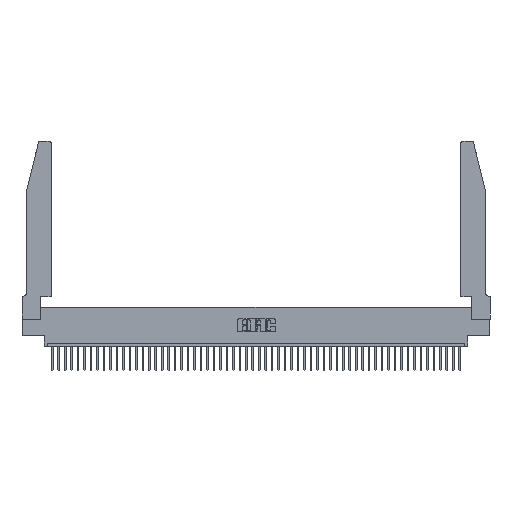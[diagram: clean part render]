
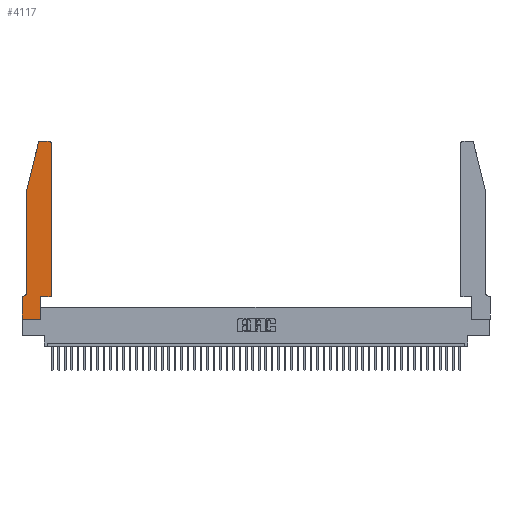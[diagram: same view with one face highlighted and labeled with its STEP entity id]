
A CAD part, top view. The second image highlights one B-rep face of the part: STEP entity #4117.
In plain terms, the highlighted planar face has unit normal (0, 0, 1).
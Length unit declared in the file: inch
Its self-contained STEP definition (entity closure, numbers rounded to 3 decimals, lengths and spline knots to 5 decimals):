
#409 = VERTEX_POINT ( 'NONE', #47005 ) ;
#2255 = CARTESIAN_POINT ( 'NONE',  ( 0.4505, 0.35, 0.37 ) ) ;
#2574 = FACE_OUTER_BOUND ( 'NONE', #24028, .T. ) ;
#3259 = CARTESIAN_POINT ( 'NONE',  ( 0.4205, 2.75, 0.37 ) ) ;
#3385 = CARTESIAN_POINT ( 'NONE',  ( 0.25487, 2.72718, 0.37 ) ) ;
#4117 = ADVANCED_FACE ( 'NONE', ( #2574 ), #21660, .T. ) ;
#5095 = ORIENTED_EDGE ( 'NONE', *, *, #29858, .T. ) ;
#5390 = ORIENTED_EDGE ( 'NONE', *, *, #9491, .T. ) ;
#6916 = ORIENTED_EDGE ( 'NONE', *, *, #14958, .T. ) ;
#8444 = VECTOR ( 'NONE', #34154, 39.37008 ) ;
#8892 = DIRECTION ( 'NONE',  ( 0., 1., 0. ) ) ;
#9297 = EDGE_CURVE ( 'NONE', #42854, #43902, #35068, .T. ) ;
#9491 = EDGE_CURVE ( 'NONE', #19205, #42175, #24732, .T. ) ;
#9789 = ORIENTED_EDGE ( 'NONE', *, *, #31108, .T. ) ;
#10030 = ORIENTED_EDGE ( 'NONE', *, *, #9297, .T. ) ;
#10309 = LINE ( 'NONE', #31914, #43622 ) ;
#10719 = VERTEX_POINT ( 'NONE', #40777 ) ;
#10902 = CARTESIAN_POINT ( 'NONE',  ( 0.284, 2.72, 0.37 ) ) ;
#12161 = LINE ( 'NONE', #43560, #28570 ) ;
#12295 = EDGE_CURVE ( 'NONE', #14741, #10719, #37264, .T. ) ;
#13896 = DIRECTION ( 'NONE',  ( -1., 0., 0. ) ) ;
#14625 = VERTEX_POINT ( 'NONE', #3385 ) ;
#14741 = VERTEX_POINT ( 'NONE', #3259 ) ;
#14958 = EDGE_CURVE ( 'NONE', #10719, #14625, #36955, .T. ) ;
#15342 = CARTESIAN_POINT ( 'NONE',  ( 0., 0., 0.37 ) ) ;
#17574 = LINE ( 'NONE', #41969, #8444 ) ;
#18045 = DIRECTION ( 'NONE',  ( 0., 0., -1. ) ) ;
#19205 = VERTEX_POINT ( 'NONE', #47621 ) ;
#19671 = CARTESIAN_POINT ( 'NONE',  ( 0.0055, 0.35, 0.37 ) ) ;
#20083 = ORIENTED_EDGE ( 'NONE', *, *, #25597, .T. ) ;
#20378 = CARTESIAN_POINT ( 'NONE',  ( 0.0755, 0.42, 0.37 ) ) ;
#21195 = ORIENTED_EDGE ( 'NONE', *, *, #40685, .T. ) ;
#21383 = CARTESIAN_POINT ( 'NONE',  ( 0.0755, 0.35, 0.37 ) ) ;
#21613 = DIRECTION ( 'NONE',  ( -1., 0., 0. ) ) ;
#21660 = PLANE ( 'NONE',  #45626 ) ;
#22224 = ORIENTED_EDGE ( 'NONE', *, *, #28083, .T. ) ;
#22719 = LINE ( 'NONE', #32537, #29141 ) ;
#23023 = EDGE_CURVE ( 'NONE', #14625, #31736, #22719, .T. ) ;
#24028 = EDGE_LOOP ( 'NONE', ( #38230, #6916, #30427, #21195, #20083, #10030, #5095, #38430, #22224, #5390, #9789, #43598 ) ) ;
#24732 = LINE ( 'NONE', #2255, #42411 ) ;
#24909 = CARTESIAN_POINT ( 'NONE',  ( 0.2865, 0.35, 0.37 ) ) ;
#25385 = DIRECTION ( 'NONE',  ( 0., 0., 1. ) ) ;
#25597 = EDGE_CURVE ( 'NONE', #33444, #42854, #49555, .T. ) ;
#25890 = AXIS2_PLACEMENT_3D ( 'NONE', #10902, #49863, #33615 ) ;
#26767 = CARTESIAN_POINT ( 'NONE',  ( 0.4505, 0.35, 0.37 ) ) ;
#28083 = EDGE_CURVE ( 'NONE', #409, #19205, #46859, .T. ) ;
#28570 = VECTOR ( 'NONE', #30235, 39.37008 ) ;
#28667 = DIRECTION ( 'NONE',  ( 0., 0., 1. ) ) ;
#28878 = EDGE_CURVE ( 'NONE', #40422, #14741, #29231, .T. ) ;
#29141 = VECTOR ( 'NONE', #32380, 39.37008 ) ;
#29231 = CIRCLE ( 'NONE', #36938, 0.03 ) ;
#29537 = CARTESIAN_POINT ( 'NONE',  ( 0.0055, 0.42, 0.37 ) ) ;
#29858 = EDGE_CURVE ( 'NONE', #43902, #39477, #12161, .T. ) ;
#29966 = VECTOR ( 'NONE', #49445, 39.37008 ) ;
#30235 = DIRECTION ( 'NONE',  ( 0., -1., 0. ) ) ;
#30427 = ORIENTED_EDGE ( 'NONE', *, *, #23023, .T. ) ;
#30443 = LINE ( 'NONE', #47049, #48540 ) ;
#31108 = EDGE_CURVE ( 'NONE', #42175, #40422, #10309, .T. ) ;
#31736 = VERTEX_POINT ( 'NONE', #37834 ) ;
#31805 = CARTESIAN_POINT ( 'NONE',  ( 0., 0.35, 0.37 ) ) ;
#31914 = CARTESIAN_POINT ( 'NONE',  ( 0.4505, 0.35, 0.37 ) ) ;
#32380 = DIRECTION ( 'NONE',  ( -0.239, -0.971, 0. ) ) ;
#32537 = CARTESIAN_POINT ( 'NONE',  ( 0.0755, 2., 0.37 ) ) ;
#32743 = DIRECTION ( 'NONE',  ( 1., 0., 0. ) ) ;
#32891 = CARTESIAN_POINT ( 'NONE',  ( 0.4205, 2.72, 0.37 ) ) ;
#33444 = VERTEX_POINT ( 'NONE', #20378 ) ;
#33615 = DIRECTION ( 'NONE',  ( 1., 0., 0. ) ) ;
#34154 = DIRECTION ( 'NONE',  ( 0., -1., 0. ) ) ;
#34763 = DIRECTION ( 'NONE',  ( 1., 0., 0. ) ) ;
#35068 = LINE ( 'NONE', #21383, #39933 ) ;
#35979 = CARTESIAN_POINT ( 'NONE',  ( 0.4505, 2.72, 0.37 ) ) ;
#35982 = VECTOR ( 'NONE', #13896, 39.37008 ) ;
#36938 = AXIS2_PLACEMENT_3D ( 'NONE', #32891, #28667, #39842 ) ;
#36955 = CIRCLE ( 'NONE', #25890, 0.03 ) ;
#37237 = DIRECTION ( 'NONE',  ( 1., 0., 0. ) ) ;
#37264 = LINE ( 'NONE', #48070, #35982 ) ;
#37834 = CARTESIAN_POINT ( 'NONE',  ( 0.0755, 2., 0.37 ) ) ;
#37912 = AXIS2_PLACEMENT_3D ( 'NONE', #29537, #18045, #38668 ) ;
#38230 = ORIENTED_EDGE ( 'NONE', *, *, #12295, .T. ) ;
#38430 = ORIENTED_EDGE ( 'NONE', *, *, #39630, .T. ) ;
#38668 = DIRECTION ( 'NONE',  ( -1., 0., 0. ) ) ;
#39477 = VERTEX_POINT ( 'NONE', #15342 ) ;
#39630 = EDGE_CURVE ( 'NONE', #39477, #409, #30443, .T. ) ;
#39842 = DIRECTION ( 'NONE',  ( 1., 0., 0. ) ) ;
#39933 = VECTOR ( 'NONE', #21613, 39.37008 ) ;
#40422 = VERTEX_POINT ( 'NONE', #35979 ) ;
#40685 = EDGE_CURVE ( 'NONE', #31736, #33444, #17574, .T. ) ;
#40777 = CARTESIAN_POINT ( 'NONE',  ( 0.284, 2.75, 0.37 ) ) ;
#41969 = CARTESIAN_POINT ( 'NONE',  ( 0.0755, 2., 0.37 ) ) ;
#42175 = VERTEX_POINT ( 'NONE', #26767 ) ;
#42411 = VECTOR ( 'NONE', #32743, 39.37008 ) ;
#42854 = VERTEX_POINT ( 'NONE', #19671 ) ;
#43560 = CARTESIAN_POINT ( 'NONE',  ( 0., 0., 0.37 ) ) ;
#43598 = ORIENTED_EDGE ( 'NONE', *, *, #28878, .T. ) ;
#43622 = VECTOR ( 'NONE', #8892, 39.37008 ) ;
#43902 = VERTEX_POINT ( 'NONE', #31805 ) ;
#45626 = AXIS2_PLACEMENT_3D ( 'NONE', #48552, #25385, #37237 ) ;
#46859 = LINE ( 'NONE', #24909, #29966 ) ;
#47005 = CARTESIAN_POINT ( 'NONE',  ( 0.2865, 0., 0.37 ) ) ;
#47049 = CARTESIAN_POINT ( 'NONE',  ( 0., 0., 0.37 ) ) ;
#47621 = CARTESIAN_POINT ( 'NONE',  ( 0.2865, 0.35, 0.37 ) ) ;
#48070 = CARTESIAN_POINT ( 'NONE',  ( 0.2605, 2.75, 0.37 ) ) ;
#48540 = VECTOR ( 'NONE', #34763, 39.37008 ) ;
#48552 = CARTESIAN_POINT ( 'NONE',  ( 0., 0.35, 0.37 ) ) ;
#49445 = DIRECTION ( 'NONE',  ( 0., 1., 0. ) ) ;
#49555 = CIRCLE ( 'NONE', #37912, 0.07 ) ;
#49863 = DIRECTION ( 'NONE',  ( 0., 0., 1. ) ) ;
